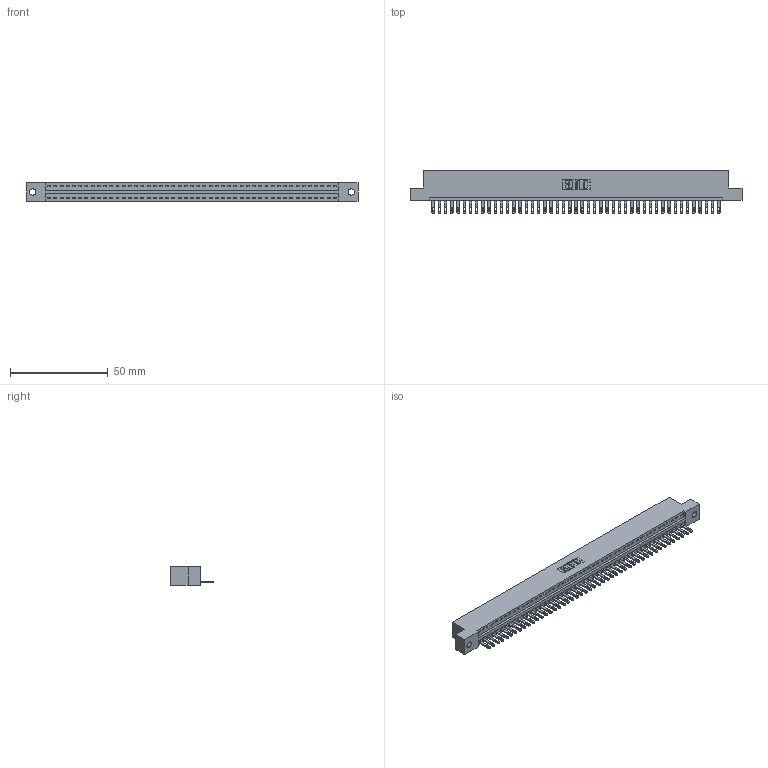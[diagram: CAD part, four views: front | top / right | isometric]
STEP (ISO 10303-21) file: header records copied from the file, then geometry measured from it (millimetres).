
FILE_DESCRIPTION (( 'STEP AP203' ), '1' );
FILE_NAME ('346-047-500-102.STEP', '2022-05-09T20:58:16', ( '' ), ( '' ), 'SwSTEP 2.0', 'SolidWorks 2020', '' );
FILE_SCHEMA (( 'CONFIG_CONTROL_DESIGN' ));
Length unit declared in the file: inch
Products named in the file (3): 346-047-500-102; 345-292-001_345-293-100; 346 Part_Flush Mounting Lugs - 0.128 Dia
Assembly tree (48 placements, depth 2):
  346-047-500-102
    346 Part_Flush Mounting Lugs - 0.128 Dia
    345-292-001_345-293-100  x47
Bounding box: 169.8 x 21.84 x 9.4 mm (x, y, z)
Volume: 16280.4 mm3; surface area: 20240.6 mm2
Topology: 48 solids, 48 shells, 2660 faces, 8225 edges, 5482 vertices
Faces by surface type: plane 1674, cylinder 986
Entity records: 28429 total; most frequent: CARTESIAN_POINT 4877, ORIENTED_EDGE 4858, DIRECTION 4299, EDGE_CURVE 2429, VECTOR 2105, LINE 2105, VERTEX_POINT 1618, AXIS2_PLACEMENT_3D 1097
